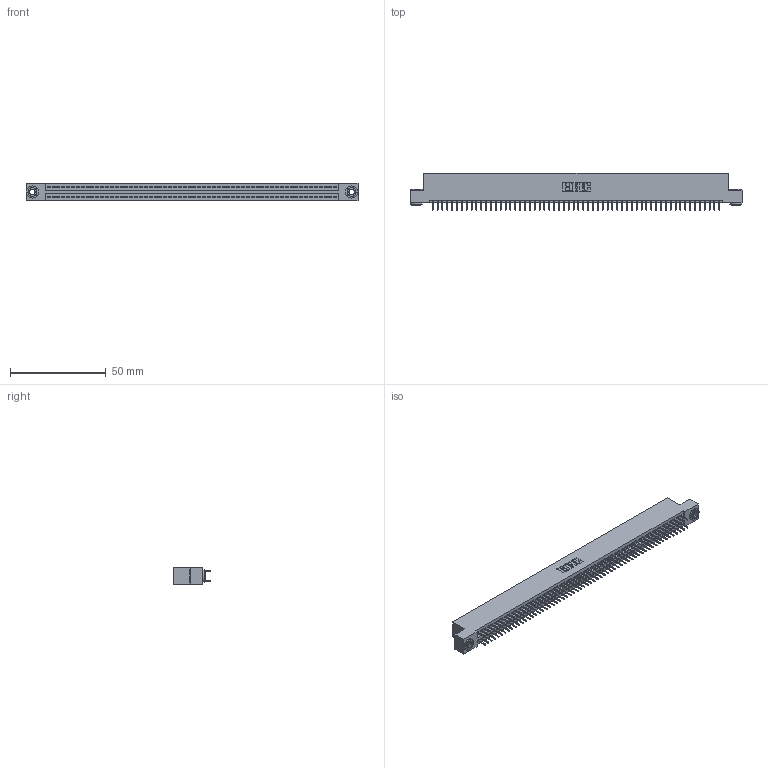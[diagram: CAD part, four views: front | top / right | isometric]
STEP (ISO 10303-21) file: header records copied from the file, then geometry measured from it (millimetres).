
FILE_DESCRIPTION (( 'STEP AP203' ), '1' );
FILE_NAME ('845-120-524-203.STEP', '2018-11-21T02:34:14', ( '' ), ( '' ), 'SwSTEP 2.0', 'SolidWorks 2016', '' );
FILE_SCHEMA (( 'CONFIG_CONTROL_DESIGN' ));
Length unit declared in the file: inch
Products named in the file (4): 845 Part_Flush Mounting Lugs - 0.156 Dia-TH; 345-292-001_345-293-124; 345-250-002_345-250-002-102; 845-120-524-203
Assembly tree (123 placements, depth 2):
  845-120-524-203
    845 Part_Flush Mounting Lugs - 0.156 Dia-TH
    345-292-001_345-293-124  x120
    345-250-002_345-250-002-102  x2
Bounding box: 173.61 x 19.35 x 9.4 mm (x, y, z)
Volume: 16869.4 mm3; surface area: 25010 mm2
Topology: 123 solids, 123 shells, 6644 faces, 18777 edges, 12034 vertices
Faces by surface type: plane 4770, cylinder 1866, cone 8
Entity records: 45378 total; most frequent: CARTESIAN_POINT 7563, ORIENTED_EDGE 7490, DIRECTION 6679, EDGE_CURVE 3745, LINE 3353, VECTOR 3353, VERTEX_POINT 2490, AXIS2_PLACEMENT_3D 1663
